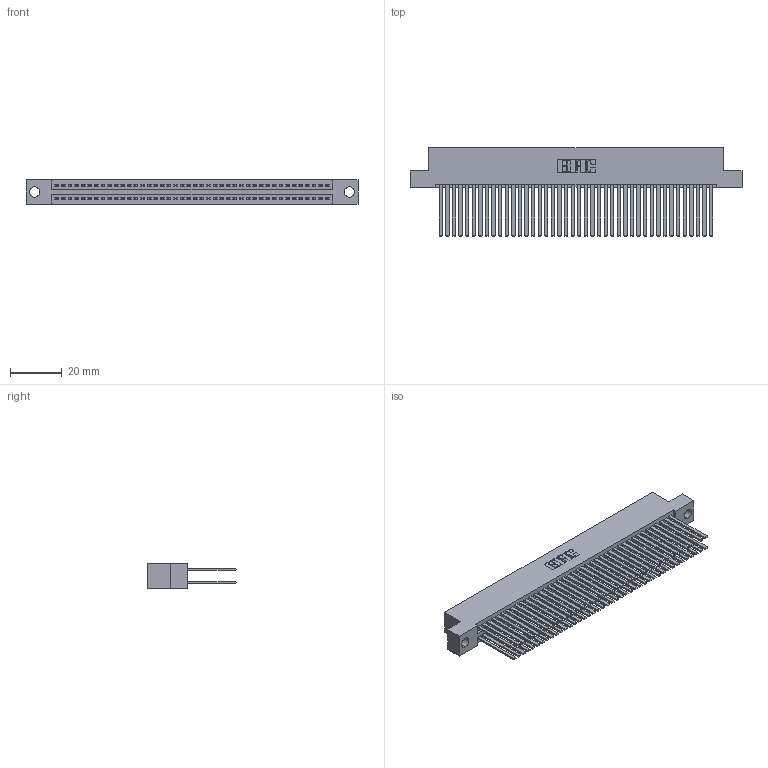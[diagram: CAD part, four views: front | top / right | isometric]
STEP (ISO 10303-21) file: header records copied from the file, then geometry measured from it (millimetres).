
FILE_DESCRIPTION (( 'STEP AP203' ), '1' );
FILE_NAME ('345-084-544-204.STEP', '2018-10-04T02:15:36', ( '' ), ( '' ), 'SwSTEP 2.0', 'SolidWorks 2016', '' );
FILE_SCHEMA (( 'CONFIG_CONTROL_DESIGN' ));
Length unit declared in the file: inch
Products named in the file (3): 345-292-001_345-293-144; 345-084-544-204; 345 Part_Flush Mounting Lugs - 0.156 Dia-TH
Assembly tree (85 placements, depth 2):
  345-084-544-204
    345 Part_Flush Mounting Lugs - 0.156 Dia-TH
    345-292-001_345-293-144  x84
Bounding box: 127.89 x 33.96 x 9.4 mm (x, y, z)
Volume: 13512.9 mm3; surface area: 23240.8 mm2
Topology: 85 solids, 85 shells, 3822 faces, 11345 edges, 7450 vertices
Faces by surface type: plane 2516, cylinder 1306
Entity records: 32773 total; most frequent: CARTESIAN_POINT 5492, ORIENTED_EDGE 5426, DIRECTION 4841, EDGE_CURVE 2713, LINE 2417, VECTOR 2417, VERTEX_POINT 1806, AXIS2_PLACEMENT_3D 1212
